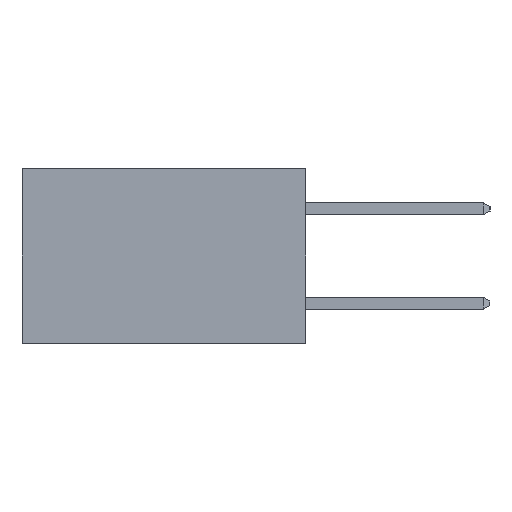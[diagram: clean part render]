
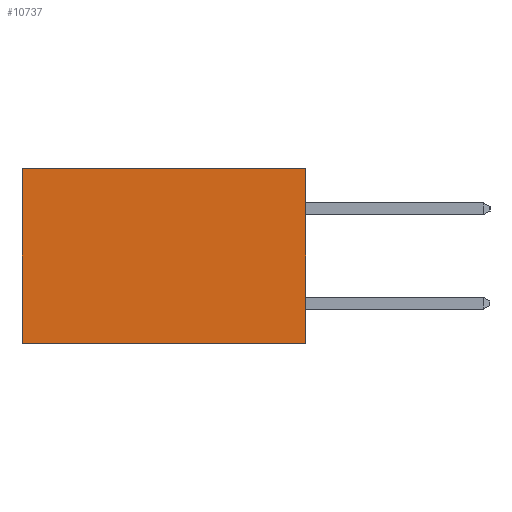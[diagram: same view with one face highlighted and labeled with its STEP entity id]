
A CAD part, left-side view. The second image highlights one B-rep face of the part: STEP entity #10737.
In plain terms, the highlighted planar face has unit normal (-1, 0, 0).
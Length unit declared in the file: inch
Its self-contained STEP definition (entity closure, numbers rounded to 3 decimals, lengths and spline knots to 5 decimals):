
#569 = DIRECTION ( 'NONE',  ( 1., 0., 0. ) ) ;
#631 = EDGE_CURVE ( 'NONE', #11610, #9216, #12973, .T. ) ;
#778 = CARTESIAN_POINT ( 'NONE',  ( 0.298, 0., 0. ) ) ;
#954 = DIRECTION ( 'NONE',  ( 0., 1., 0. ) ) ;
#1086 = ORIENTED_EDGE ( 'NONE', *, *, #631, .T. ) ;
#1123 = EDGE_CURVE ( 'NONE', #11610, #15187, #3174, .T. ) ;
#1278 = EDGE_CURVE ( 'NONE', #15187, #5612, #8224, .T. ) ;
#1288 = CARTESIAN_POINT ( 'NONE',  ( 0.298, 0., -0.37 ) ) ;
#3174 = LINE ( 'NONE', #11664, #17461 ) ;
#3590 = LINE ( 'NONE', #13540, #17439 ) ;
#3992 = ORIENTED_EDGE ( 'NONE', *, *, #5744, .T. ) ;
#4654 = VECTOR ( 'NONE', #8219, 39.37008 ) ;
#5612 = VERTEX_POINT ( 'NONE', #16264 ) ;
#5735 = VECTOR ( 'NONE', #954, 39.37008 ) ;
#5744 = EDGE_CURVE ( 'NONE', #9216, #5612, #3590, .T. ) ;
#7070 = CARTESIAN_POINT ( 'NONE',  ( 0.298, 0.6, 0. ) ) ;
#8156 = EDGE_LOOP ( 'NONE', ( #3992, #15735, #15970, #1086 ) ) ;
#8219 = DIRECTION ( 'NONE',  ( 0., 1., 0. ) ) ;
#8224 = LINE ( 'NONE', #1288, #4654 ) ;
#9216 = VERTEX_POINT ( 'NONE', #7070 ) ;
#9454 = DIRECTION ( 'NONE',  ( 0., 0., -1. ) ) ;
#9462 = FACE_OUTER_BOUND ( 'NONE', #8156, .T. ) ;
#10029 = DIRECTION ( 'NONE',  ( 0., 0., -1. ) ) ;
#10737 = ADVANCED_FACE ( 'NONE', ( #9462 ), #15473, .F. ) ;
#11091 = DIRECTION ( 'NONE',  ( 0., 0., -1. ) ) ;
#11610 = VERTEX_POINT ( 'NONE', #13060 ) ;
#11664 = CARTESIAN_POINT ( 'NONE',  ( 0.298, 0., 0. ) ) ;
#12723 = AXIS2_PLACEMENT_3D ( 'NONE', #12754, #569, #10029 ) ;
#12754 = CARTESIAN_POINT ( 'NONE',  ( 0.298, 0., 0. ) ) ;
#12973 = LINE ( 'NONE', #778, #5735 ) ;
#13060 = CARTESIAN_POINT ( 'NONE',  ( 0.298, 0., 0. ) ) ;
#13540 = CARTESIAN_POINT ( 'NONE',  ( 0.298, 0.6, 0. ) ) ;
#15086 = CARTESIAN_POINT ( 'NONE',  ( 0.298, 0., -0.37 ) ) ;
#15187 = VERTEX_POINT ( 'NONE', #15086 ) ;
#15473 = PLANE ( 'NONE',  #12723 ) ;
#15735 = ORIENTED_EDGE ( 'NONE', *, *, #1278, .F. ) ;
#15970 = ORIENTED_EDGE ( 'NONE', *, *, #1123, .F. ) ;
#16264 = CARTESIAN_POINT ( 'NONE',  ( 0.298, 0.6, -0.37 ) ) ;
#17439 = VECTOR ( 'NONE', #9454, 39.37008 ) ;
#17461 = VECTOR ( 'NONE', #11091, 39.37008 ) ;
